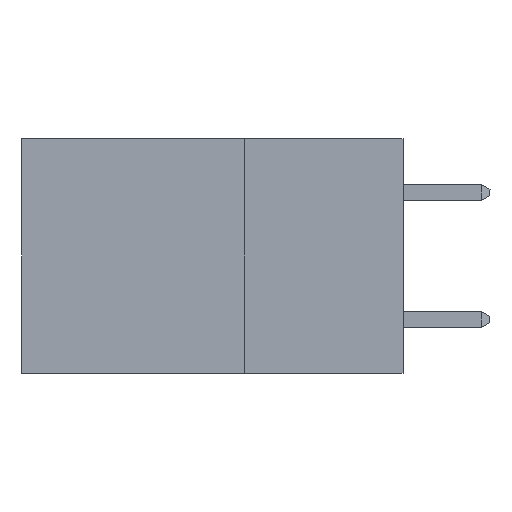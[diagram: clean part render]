
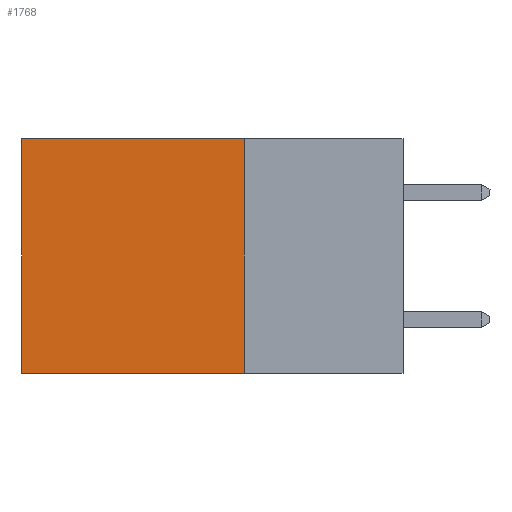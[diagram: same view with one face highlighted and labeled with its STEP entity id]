
A CAD part, left-side view. The second image highlights one B-rep face of the part: STEP entity #1768.
In plain terms, the highlighted planar face has unit normal (-1, 0, 0).
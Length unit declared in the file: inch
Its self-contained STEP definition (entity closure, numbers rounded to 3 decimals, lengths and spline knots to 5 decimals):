
#14 = PLANE ( 'NONE',  #3306 ) ;
#133 = CARTESIAN_POINT ( 'NONE',  ( 0.2875, 0.25, -0.37 ) ) ;
#187 = ORIENTED_EDGE ( 'NONE', *, *, #8655, .F. ) ;
#387 = LINE ( 'NONE', #7796, #2468 ) ;
#389 = VERTEX_POINT ( 'NONE', #133 ) ;
#898 = ORIENTED_EDGE ( 'NONE', *, *, #5054, .F. ) ;
#1768 = ADVANCED_FACE ( 'NONE', ( #8783 ), #14, .F. ) ;
#2243 = DIRECTION ( 'NONE',  ( 0., 0., -1. ) ) ;
#2308 = CARTESIAN_POINT ( 'NONE',  ( 0.2875, 0.25, 0. ) ) ;
#2468 = VECTOR ( 'NONE', #10384, 39.37008 ) ;
#3261 = CARTESIAN_POINT ( 'NONE',  ( 0.2875, 0.25, 0. ) ) ;
#3306 = AXIS2_PLACEMENT_3D ( 'NONE', #10820, #9768, #8961 ) ;
#3396 = CARTESIAN_POINT ( 'NONE',  ( 0.2875, 0.25, -0.37 ) ) ;
#3865 = ORIENTED_EDGE ( 'NONE', *, *, #6924, .T. ) ;
#4512 = EDGE_LOOP ( 'NONE', ( #7388, #898, #187, #3865 ) ) ;
#5054 = EDGE_CURVE ( 'NONE', #389, #10691, #6344, .T. ) ;
#5128 = DIRECTION ( 'NONE',  ( 0., 1., 0. ) ) ;
#5462 = VECTOR ( 'NONE', #2243, 39.37008 ) ;
#6344 = LINE ( 'NONE', #3396, #10285 ) ;
#6497 = CARTESIAN_POINT ( 'NONE',  ( 0.2875, 0.6, 0. ) ) ;
#6542 = VERTEX_POINT ( 'NONE', #9255 ) ;
#6924 = EDGE_CURVE ( 'NONE', #10065, #6542, #387, .T. ) ;
#7388 = ORIENTED_EDGE ( 'NONE', *, *, #11141, .T. ) ;
#7410 = DIRECTION ( 'NONE',  ( 0., 0., -1. ) ) ;
#7796 = CARTESIAN_POINT ( 'NONE',  ( 0.2875, 0.25, 0. ) ) ;
#8655 = EDGE_CURVE ( 'NONE', #10065, #389, #10255, .T. ) ;
#8783 = FACE_OUTER_BOUND ( 'NONE', #4512, .T. ) ;
#8961 = DIRECTION ( 'NONE',  ( 0., 0., -1. ) ) ;
#9255 = CARTESIAN_POINT ( 'NONE',  ( 0.2875, 0.6, 0. ) ) ;
#9345 = LINE ( 'NONE', #6497, #11474 ) ;
#9768 = DIRECTION ( 'NONE',  ( 1., 0., 0. ) ) ;
#10065 = VERTEX_POINT ( 'NONE', #3261 ) ;
#10255 = LINE ( 'NONE', #2308, #5462 ) ;
#10285 = VECTOR ( 'NONE', #5128, 39.37008 ) ;
#10384 = DIRECTION ( 'NONE',  ( 0., 1., 0. ) ) ;
#10691 = VERTEX_POINT ( 'NONE', #11395 ) ;
#10820 = CARTESIAN_POINT ( 'NONE',  ( 0.2875, 0.25, 0. ) ) ;
#11141 = EDGE_CURVE ( 'NONE', #6542, #10691, #9345, .T. ) ;
#11395 = CARTESIAN_POINT ( 'NONE',  ( 0.2875, 0.6, -0.37 ) ) ;
#11474 = VECTOR ( 'NONE', #7410, 39.37008 ) ;
